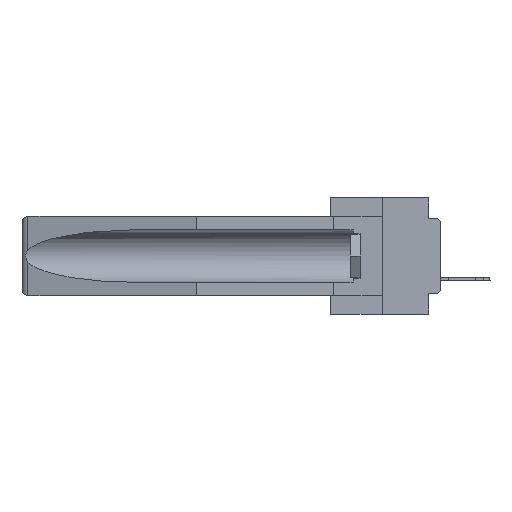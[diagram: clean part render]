
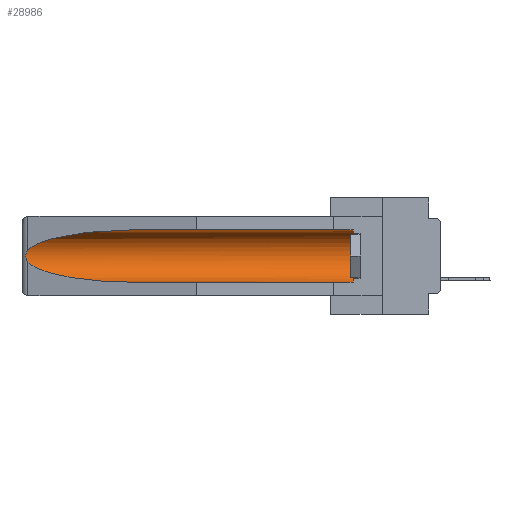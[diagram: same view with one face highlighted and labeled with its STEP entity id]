
A CAD part, left-side view. The second image highlights one B-rep face of the part: STEP entity #28986.
In plain terms, the highlighted cylindrical face has radius 2.857 mm (diameter 5.715 mm), a partial arc.
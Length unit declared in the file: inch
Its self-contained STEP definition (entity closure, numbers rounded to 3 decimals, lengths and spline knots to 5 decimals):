
#10 = LINE ( 'NONE', #2713, #28312 ) ;
#2713 = CARTESIAN_POINT ( 'NONE',  ( 0.155, -0.30754, -0.059 ) ) ;
#2905 = CARTESIAN_POINT ( 'NONE',  ( 0.25451, 1.48313, -0.24835 ) ) ;
#4287 = ORIENTED_EDGE ( 'NONE', *, *, #20162, .T. ) ;
#4569 = EDGE_CURVE ( 'NONE', #11661, #38178, #22029, .T. ) ;
#4642 = VERTEX_POINT ( 'NONE', #20594 ) ;
#5011 = CARTESIAN_POINT ( 'NONE',  ( 0.26597, 1.52961, -0.15275 ) ) ;
#5143 = CARTESIAN_POINT ( 'NONE',  ( 0.2675, 1.53308, -0.16763 ) ) ;
#5526 = VERTEX_POINT ( 'NONE', #13525 ) ;
#5789 = ORIENTED_EDGE ( 'NONE', *, *, #4569, .T. ) ;
#6209 = DIRECTION ( 'NONE',  ( 0., -1., 0. ) ) ;
#8218 = CARTESIAN_POINT ( 'NONE',  ( 0.26597, 1.5296, -0.19026 ) ) ;
#8756 = DIRECTION ( 'NONE',  ( 0., 0., 1. ) ) ;
#9423 = B_SPLINE_CURVE_WITH_KNOTS ( 'NONE', 3,
 ( #37750, #5011, #16569, #10970, #5143, #26024, #31340, #22896, #8218, #19912 ),
 .UNSPECIFIED., .F., .F.,
 ( 4, 2, 2, 2, 4 ),
 ( 0., 0.00029, 0.00058, 0.00087, 0.00117 ),
 .UNSPECIFIED. ) ;
#10609 =( BOUNDED_CURVE ( )  B_SPLINE_CURVE ( 3, ( #14673, #2905, #29948, #20629 ),
 .UNSPECIFIED., .F., .F. ) 
 B_SPLINE_CURVE_WITH_KNOTS ( ( 4, 4 ),
 ( 0.1948, 1.5708 ),
 .UNSPECIFIED. ) 
 CURVE ( )  GEOMETRIC_REPRESENTATION_ITEM ( )  RATIONAL_B_SPLINE_CURVE ( ( 1., 0.848, 0.848, 1. ) ) 
 REPRESENTATION_ITEM ( '' )  );
#10970 = CARTESIAN_POINT ( 'NONE',  ( 0.2673, 1.5327, -0.16383 ) ) ;
#11661 = VERTEX_POINT ( 'NONE', #36053 ) ;
#11665 = EDGE_CURVE ( 'NONE', #5526, #33486, #24948, .T. ) ;
#12478 = CARTESIAN_POINT ( 'NONE',  ( 0.155, 1.07973, -0.284 ) ) ;
#13525 = CARTESIAN_POINT ( 'NONE',  ( 0.155, 0.126, -0.284 ) ) ;
#13631 = EDGE_CURVE ( 'NONE', #38178, #4642, #9423, .T. ) ;
#14130 = CARTESIAN_POINT ( 'NONE',  ( 0.155, 1.07973, -0.059 ) ) ;
#14673 = CARTESIAN_POINT ( 'NONE',  ( 0.26537, 1.52718, -0.19328 ) ) ;
#15178 = ORIENTED_EDGE ( 'NONE', *, *, #13631, .T. ) ;
#16294 = CARTESIAN_POINT ( 'NONE',  ( 0.26537, 1.52718, -0.14972 ) ) ;
#16569 = CARTESIAN_POINT ( 'NONE',  ( 0.26654, 1.53092, -0.15636 ) ) ;
#16827 = AXIS2_PLACEMENT_3D ( 'NONE', #22420, #22548, #28254 ) ;
#18300 = DIRECTION ( 'NONE',  ( 0., 1., 0. ) ) ;
#19912 = CARTESIAN_POINT ( 'NONE',  ( 0.26537, 1.52718, -0.19328 ) ) ;
#20162 = EDGE_CURVE ( 'NONE', #5526, #36868, #27807, .T. ) ;
#20293 = VECTOR ( 'NONE', #18300, 39.37008 ) ;
#20594 = CARTESIAN_POINT ( 'NONE',  ( 0.26537, 1.52718, -0.19328 ) ) ;
#20629 = CARTESIAN_POINT ( 'NONE',  ( 0.155, 1.07973, -0.284 ) ) ;
#20707 = EDGE_CURVE ( 'NONE', #4642, #33486, #10609, .T. ) ;
#20726 = CARTESIAN_POINT ( 'NONE',  ( 0.155, -0.30754, -0.284 ) ) ;
#22029 =( BOUNDED_CURVE ( )  B_SPLINE_CURVE ( 3, ( #14130, #35270, #32165, #23313 ),
 .UNSPECIFIED., .F., .T. ) 
 B_SPLINE_CURVE_WITH_KNOTS ( ( 4, 4 ),
 ( 4.71239, 6.08839 ),
 .UNSPECIFIED. ) 
 CURVE ( )  GEOMETRIC_REPRESENTATION_ITEM ( )  RATIONAL_B_SPLINE_CURVE ( ( 1., 0.848, 0.848, 1. ) ) 
 REPRESENTATION_ITEM ( '' )  );
#22420 = CARTESIAN_POINT ( 'NONE',  ( 0.155, -0.30754, -0.1715 ) ) ;
#22522 = AXIS2_PLACEMENT_3D ( 'NONE', #26439, #6209, #8756 ) ;
#22548 = DIRECTION ( 'NONE',  ( 0., 1., 0. ) ) ;
#22896 = CARTESIAN_POINT ( 'NONE',  ( 0.26655, 1.53094, -0.18657 ) ) ;
#23313 = CARTESIAN_POINT ( 'NONE',  ( 0.26537, 1.52718, -0.14972 ) ) ;
#23632 = CYLINDRICAL_SURFACE ( 'NONE', #16827, 0.1125 ) ;
#23939 = ORIENTED_EDGE ( 'NONE', *, *, #20707, .T. ) ;
#24948 = LINE ( 'NONE', #20726, #20293 ) ;
#26024 = CARTESIAN_POINT ( 'NONE',  ( 0.2675, 1.53308, -0.17534 ) ) ;
#26193 = DIRECTION ( 'NONE',  ( 0., 1., 0. ) ) ;
#26439 = CARTESIAN_POINT ( 'NONE',  ( 0.155, 0.126, -0.1715 ) ) ;
#27807 = CIRCLE ( 'NONE', #22522, 0.1125 ) ;
#27838 = FACE_OUTER_BOUND ( 'NONE', #30600, .T. ) ;
#28050 = CARTESIAN_POINT ( 'NONE',  ( 0.155, 0.126, -0.059 ) ) ;
#28254 = DIRECTION ( 'NONE',  ( 0., 0., 1. ) ) ;
#28312 = VECTOR ( 'NONE', #26193, 39.37008 ) ;
#28986 = ADVANCED_FACE ( 'NONE', ( #27838 ), #23632, .F. ) ;
#29310 = ORIENTED_EDGE ( 'NONE', *, *, #37463, .T. ) ;
#29948 = CARTESIAN_POINT ( 'NONE',  ( 0.21114, 1.30732, -0.284 ) ) ;
#30600 = EDGE_LOOP ( 'NONE', ( #5789, #15178, #23939, #33616, #4287, #29310 ) ) ;
#31340 = CARTESIAN_POINT ( 'NONE',  ( 0.2673, 1.53269, -0.17917 ) ) ;
#32165 = CARTESIAN_POINT ( 'NONE',  ( 0.25451, 1.48313, -0.09465 ) ) ;
#33486 = VERTEX_POINT ( 'NONE', #12478 ) ;
#33616 = ORIENTED_EDGE ( 'NONE', *, *, #11665, .F. ) ;
#35270 = CARTESIAN_POINT ( 'NONE',  ( 0.21114, 1.30732, -0.059 ) ) ;
#36053 = CARTESIAN_POINT ( 'NONE',  ( 0.155, 1.07973, -0.059 ) ) ;
#36868 = VERTEX_POINT ( 'NONE', #28050 ) ;
#37463 = EDGE_CURVE ( 'NONE', #36868, #11661, #10, .T. ) ;
#37750 = CARTESIAN_POINT ( 'NONE',  ( 0.26537, 1.52718, -0.14972 ) ) ;
#38178 = VERTEX_POINT ( 'NONE', #16294 ) ;
